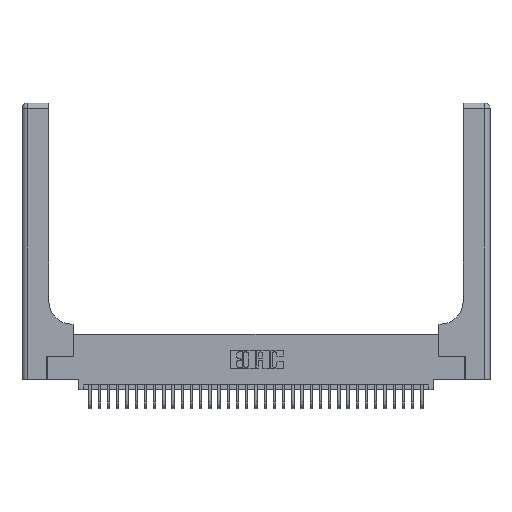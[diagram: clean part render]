
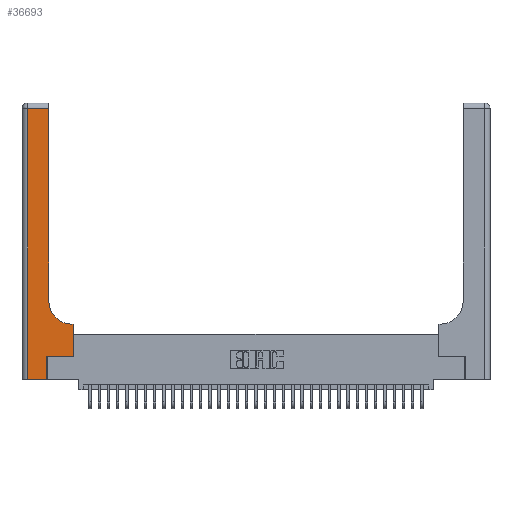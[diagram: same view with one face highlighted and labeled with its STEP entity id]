
A CAD part, top view. The second image highlights one B-rep face of the part: STEP entity #36693.
In plain terms, the highlighted planar face has unit normal (0, 0, 1).
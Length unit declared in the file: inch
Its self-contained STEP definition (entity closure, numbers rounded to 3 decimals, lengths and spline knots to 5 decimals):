
#91 = EDGE_LOOP ( 'NONE', ( #6381, #24606, #23852, #9241, #24365, #16587, #13068, #15598, #9421 ) ) ;
#501 = VERTEX_POINT ( 'NONE', #12806 ) ;
#897 = VECTOR ( 'NONE', #1395, 39.37008 ) ;
#1395 = DIRECTION ( 'NONE',  ( 0., -1., 0. ) ) ;
#1849 = VECTOR ( 'NONE', #16582, 39.37008 ) ;
#1858 = CARTESIAN_POINT ( 'NONE',  ( 0.269, 0., 0.37 ) ) ;
#2574 = CARTESIAN_POINT ( 'NONE',  ( 0.2915, 2.94, 0.37 ) ) ;
#2801 = EDGE_CURVE ( 'NONE', #9457, #9344, #8447, .T. ) ;
#3158 = LINE ( 'NONE', #1858, #24042 ) ;
#3449 = VERTEX_POINT ( 'NONE', #21168 ) ;
#3946 = CARTESIAN_POINT ( 'NONE',  ( 0., 3., 0.37 ) ) ;
#4899 = CARTESIAN_POINT ( 'NONE',  ( 0.5585, 0.25, 0.37 ) ) ;
#5503 = VECTOR ( 'NONE', #29055, 39.37008 ) ;
#5772 = LINE ( 'NONE', #9446, #27478 ) ;
#6381 = ORIENTED_EDGE ( 'NONE', *, *, #26047, .T. ) ;
#6823 = DIRECTION ( 'NONE',  ( 0., 0., -1. ) ) ;
#7063 = CARTESIAN_POINT ( 'NONE',  ( 0.06, 0., 0.37 ) ) ;
#7409 = CARTESIAN_POINT ( 'NONE',  ( 0.2915, 3., 0.37 ) ) ;
#8447 = LINE ( 'NONE', #15393, #15128 ) ;
#8804 = DIRECTION ( 'NONE',  ( 0., 0., -1. ) ) ;
#8987 = CARTESIAN_POINT ( 'NONE',  ( 0.2915, 0.85, 0.37 ) ) ;
#9241 = ORIENTED_EDGE ( 'NONE', *, *, #2801, .T. ) ;
#9321 = EDGE_CURVE ( 'NONE', #14481, #34555, #13955, .T. ) ;
#9344 = VERTEX_POINT ( 'NONE', #32057 ) ;
#9421 = ORIENTED_EDGE ( 'NONE', *, *, #28749, .T. ) ;
#9446 = CARTESIAN_POINT ( 'NONE',  ( 0.2915, 0.6, 0.37 ) ) ;
#9457 = VERTEX_POINT ( 'NONE', #7063 ) ;
#10326 = VERTEX_POINT ( 'NONE', #36446 ) ;
#12094 = LINE ( 'NONE', #7409, #25384 ) ;
#12546 = DIRECTION ( 'NONE',  ( 1., 0., 0. ) ) ;
#12781 = CARTESIAN_POINT ( 'NONE',  ( 0.06, 2.94, 0.37 ) ) ;
#12806 = CARTESIAN_POINT ( 'NONE',  ( 0.5585, 0.6, 0.37 ) ) ;
#13068 = ORIENTED_EDGE ( 'NONE', *, *, #31741, .T. ) ;
#13719 = CARTESIAN_POINT ( 'NONE',  ( 0.269, 0.25, 0.37 ) ) ;
#13955 = LINE ( 'NONE', #31936, #5503 ) ;
#14481 = VERTEX_POINT ( 'NONE', #2574 ) ;
#15128 = VECTOR ( 'NONE', #12546, 39.37008 ) ;
#15393 = CARTESIAN_POINT ( 'NONE',  ( 0., 0., 0.37 ) ) ;
#15598 = ORIENTED_EDGE ( 'NONE', *, *, #30255, .T. ) ;
#16200 = AXIS2_PLACEMENT_3D ( 'NONE', #3946, #6823, #26608 ) ;
#16310 = AXIS2_PLACEMENT_3D ( 'NONE', #25752, #8804, #28575 ) ;
#16582 = DIRECTION ( 'NONE',  ( 1., 0., 0. ) ) ;
#16587 = ORIENTED_EDGE ( 'NONE', *, *, #26193, .T. ) ;
#16873 = VERTEX_POINT ( 'NONE', #8987 ) ;
#17509 = VERTEX_POINT ( 'NONE', #19120 ) ;
#18892 = DIRECTION ( 'NONE',  ( 0., 1., 0. ) ) ;
#19120 = CARTESIAN_POINT ( 'NONE',  ( 0.5415, 0.6, 0.37 ) ) ;
#19960 = CIRCLE ( 'NONE', #16310, 0.25 ) ;
#21168 = CARTESIAN_POINT ( 'NONE',  ( 0.269, 0.25, 0.37 ) ) ;
#23852 = ORIENTED_EDGE ( 'NONE', *, *, #29680, .T. ) ;
#24042 = VECTOR ( 'NONE', #18892, 39.37008 ) ;
#24365 = ORIENTED_EDGE ( 'NONE', *, *, #36295, .T. ) ;
#24385 = DIRECTION ( 'NONE',  ( 0., 1., 0. ) ) ;
#24606 = ORIENTED_EDGE ( 'NONE', *, *, #9321, .T. ) ;
#24759 = VECTOR ( 'NONE', #30253, 39.37008 ) ;
#24915 = FACE_OUTER_BOUND ( 'NONE', #91, .T. ) ;
#25384 = VECTOR ( 'NONE', #24385, 39.37008 ) ;
#25608 = LINE ( 'NONE', #4899, #24759 ) ;
#25752 = CARTESIAN_POINT ( 'NONE',  ( 0.5415, 0.85, 0.37 ) ) ;
#26047 = EDGE_CURVE ( 'NONE', #16873, #14481, #12094, .T. ) ;
#26193 = EDGE_CURVE ( 'NONE', #3449, #10326, #35993, .T. ) ;
#26388 = DIRECTION ( 'NONE',  ( -1., 0., 0. ) ) ;
#26608 = DIRECTION ( 'NONE',  ( -1., 0., 0. ) ) ;
#27478 = VECTOR ( 'NONE', #26388, 39.37008 ) ;
#28575 = DIRECTION ( 'NONE',  ( 1., 0., 0. ) ) ;
#28749 = EDGE_CURVE ( 'NONE', #17509, #16873, #19960, .T. ) ;
#29055 = DIRECTION ( 'NONE',  ( -1., 0., 0. ) ) ;
#29680 = EDGE_CURVE ( 'NONE', #34555, #9457, #31050, .T. ) ;
#29748 = CARTESIAN_POINT ( 'NONE',  ( 0.06, 3., 0.37 ) ) ;
#30253 = DIRECTION ( 'NONE',  ( 0., 1., 0. ) ) ;
#30255 = EDGE_CURVE ( 'NONE', #501, #17509, #5772, .T. ) ;
#31050 = LINE ( 'NONE', #29748, #897 ) ;
#31741 = EDGE_CURVE ( 'NONE', #10326, #501, #25608, .T. ) ;
#31936 = CARTESIAN_POINT ( 'NONE',  ( 0., 2.94, 0.37 ) ) ;
#32057 = CARTESIAN_POINT ( 'NONE',  ( 0.269, 0., 0.37 ) ) ;
#32188 = PLANE ( 'NONE',  #16200 ) ;
#34555 = VERTEX_POINT ( 'NONE', #12781 ) ;
#35993 = LINE ( 'NONE', #13719, #1849 ) ;
#36295 = EDGE_CURVE ( 'NONE', #9344, #3449, #3158, .T. ) ;
#36446 = CARTESIAN_POINT ( 'NONE',  ( 0.5585, 0.25, 0.37 ) ) ;
#36693 = ADVANCED_FACE ( 'NONE', ( #24915 ), #32188, .F. ) ;
